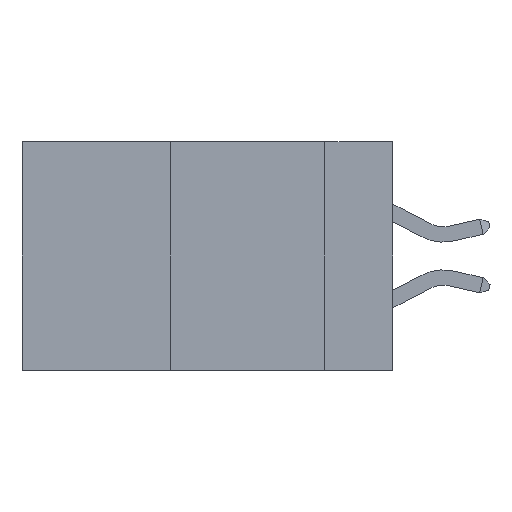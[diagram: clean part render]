
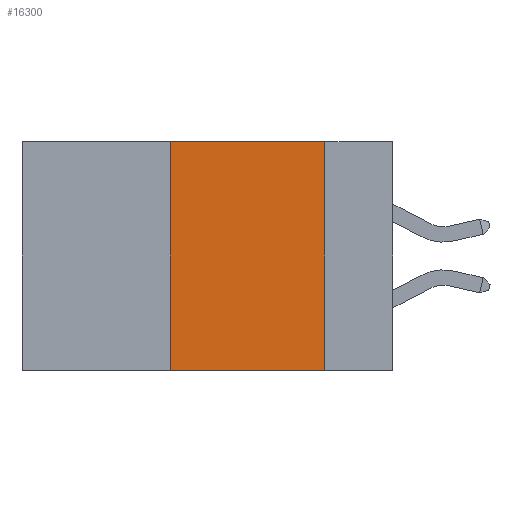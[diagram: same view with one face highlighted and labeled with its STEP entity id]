
A CAD part, left-side view. The second image highlights one B-rep face of the part: STEP entity #16300.
In plain terms, the highlighted planar face has unit normal (-1, 0, 0).
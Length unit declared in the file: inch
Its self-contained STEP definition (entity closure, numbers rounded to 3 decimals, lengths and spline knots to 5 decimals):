
#123 = EDGE_LOOP ( 'NONE', ( #19536, #19123, #14075, #17574 ) ) ;
#574 = CARTESIAN_POINT ( 'NONE',  ( 0., 0.6, 0. ) ) ;
#750 = LINE ( 'NONE', #14731, #19982 ) ;
#2281 = CARTESIAN_POINT ( 'NONE',  ( 0., 0.36, 0. ) ) ;
#2903 = DIRECTION ( 'NONE',  ( 0., -1., 0. ) ) ;
#3597 = VERTEX_POINT ( 'NONE', #19557 ) ;
#3814 = CARTESIAN_POINT ( 'NONE',  ( 0., 0.11, -0.37 ) ) ;
#3924 = DIRECTION ( 'NONE',  ( 1., 0., 0. ) ) ;
#4423 = VERTEX_POINT ( 'NONE', #3814 ) ;
#4834 = LINE ( 'NONE', #15966, #20370 ) ;
#5697 = LINE ( 'NONE', #5853, #17334 ) ;
#5853 = CARTESIAN_POINT ( 'NONE',  ( 0., 0.6, -0.37 ) ) ;
#6912 = CARTESIAN_POINT ( 'NONE',  ( 0., 0.36, 0. ) ) ;
#7603 = PLANE ( 'NONE',  #18055 ) ;
#8790 = CARTESIAN_POINT ( 'NONE',  ( 0., 0.11, 0. ) ) ;
#9838 = EDGE_CURVE ( 'NONE', #10097, #4423, #750, .T. ) ;
#10097 = VERTEX_POINT ( 'NONE', #8790 ) ;
#11572 = LINE ( 'NONE', #2281, #20625 ) ;
#13778 = EDGE_CURVE ( 'NONE', #21356, #10097, #4834, .T. ) ;
#13958 = DIRECTION ( 'NONE',  ( 0., -1., 0. ) ) ;
#13984 = EDGE_CURVE ( 'NONE', #3597, #21356, #11572, .T. ) ;
#14075 = ORIENTED_EDGE ( 'NONE', *, *, #13984, .F. ) ;
#14327 = FACE_OUTER_BOUND ( 'NONE', #123, .T. ) ;
#14731 = CARTESIAN_POINT ( 'NONE',  ( 0., 0.11, 0. ) ) ;
#15966 = CARTESIAN_POINT ( 'NONE',  ( 0., 0.6, 0. ) ) ;
#16300 = ADVANCED_FACE ( 'NONE', ( #14327 ), #7603, .F. ) ;
#17334 = VECTOR ( 'NONE', #13958, 39.37008 ) ;
#17574 = ORIENTED_EDGE ( 'NONE', *, *, #17996, .T. ) ;
#17950 = DIRECTION ( 'NONE',  ( 0., 0., -1. ) ) ;
#17996 = EDGE_CURVE ( 'NONE', #3597, #4423, #5697, .T. ) ;
#18055 = AXIS2_PLACEMENT_3D ( 'NONE', #574, #3924, #18866 ) ;
#18866 = DIRECTION ( 'NONE',  ( 0., 0., -1. ) ) ;
#19123 = ORIENTED_EDGE ( 'NONE', *, *, #13778, .F. ) ;
#19256 = DIRECTION ( 'NONE',  ( 0., 0., 1. ) ) ;
#19536 = ORIENTED_EDGE ( 'NONE', *, *, #9838, .F. ) ;
#19557 = CARTESIAN_POINT ( 'NONE',  ( 0., 0.36, -0.37 ) ) ;
#19982 = VECTOR ( 'NONE', #17950, 39.37008 ) ;
#20370 = VECTOR ( 'NONE', #2903, 39.37008 ) ;
#20625 = VECTOR ( 'NONE', #19256, 39.37008 ) ;
#21356 = VERTEX_POINT ( 'NONE', #6912 ) ;
